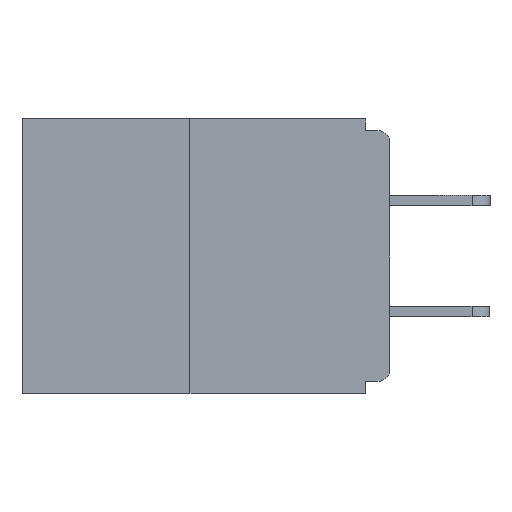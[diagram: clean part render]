
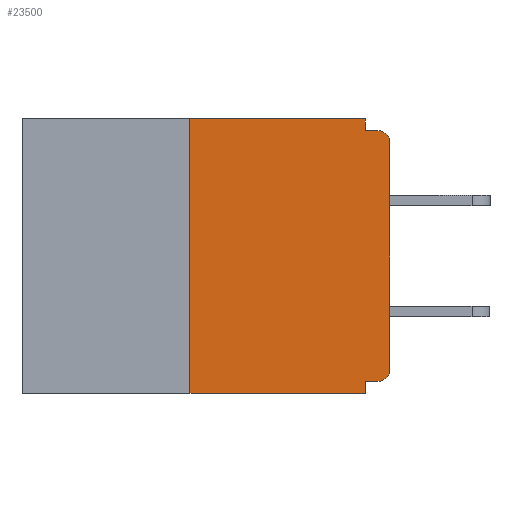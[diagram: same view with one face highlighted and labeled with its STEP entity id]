
A CAD part, left-side view. The second image highlights one B-rep face of the part: STEP entity #23500.
In plain terms, the highlighted planar face has unit normal (-1, 0, 0).
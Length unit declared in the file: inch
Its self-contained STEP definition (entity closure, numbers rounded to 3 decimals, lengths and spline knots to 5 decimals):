
#420 = DIRECTION ( 'NONE',  ( 0., 0., -1. ) ) ;
#530 = AXIS2_PLACEMENT_3D ( 'NONE', #22053, #16932, #420 ) ;
#703 = CARTESIAN_POINT ( 'NONE',  ( 0., 0.015, -0.015 ) ) ;
#951 = DIRECTION ( 'NONE',  ( -1., 0., 0. ) ) ;
#2129 = LINE ( 'NONE', #2693, #16159 ) ;
#2439 = CARTESIAN_POINT ( 'NONE',  ( 0., 0.015, -0.328 ) ) ;
#2693 = CARTESIAN_POINT ( 'NONE',  ( 0., 0.031, 0. ) ) ;
#3044 = EDGE_CURVE ( 'NONE', #8765, #3837, #5856, .T. ) ;
#3158 = LINE ( 'NONE', #17375, #16591 ) ;
#3267 = VERTEX_POINT ( 'NONE', #6853 ) ;
#3383 = CARTESIAN_POINT ( 'NONE',  ( 0., 0., -0.015 ) ) ;
#3719 = CARTESIAN_POINT ( 'NONE',  ( 0., 0.46, -0.343 ) ) ;
#3837 = VERTEX_POINT ( 'NONE', #6579 ) ;
#3854 = EDGE_CURVE ( 'NONE', #17910, #6839, #3158, .T. ) ;
#3873 = FACE_OUTER_BOUND ( 'NONE', #7783, .T. ) ;
#3999 = PLANE ( 'NONE',  #530 ) ;
#4750 = CARTESIAN_POINT ( 'NONE',  ( 0., 0.46, 0. ) ) ;
#5240 = EDGE_CURVE ( 'NONE', #3267, #11360, #7629, .T. ) ;
#5808 = DIRECTION ( 'NONE',  ( 0., -1., 0. ) ) ;
#5856 = CIRCLE ( 'NONE', #20190, 0.015 ) ;
#5893 = ORIENTED_EDGE ( 'NONE', *, *, #5240, .F. ) ;
#6246 = ORIENTED_EDGE ( 'NONE', *, *, #3854, .F. ) ;
#6266 = VERTEX_POINT ( 'NONE', #19514 ) ;
#6411 = DIRECTION ( 'NONE',  ( 0., 0., 1. ) ) ;
#6579 = CARTESIAN_POINT ( 'NONE',  ( 0., 0., -0.313 ) ) ;
#6693 = VECTOR ( 'NONE', #16427, 39.37008 ) ;
#6839 = VERTEX_POINT ( 'NONE', #11793 ) ;
#6853 = CARTESIAN_POINT ( 'NONE',  ( 0., 0.031, -0.328 ) ) ;
#7018 = ORIENTED_EDGE ( 'NONE', *, *, #14868, .F. ) ;
#7549 = VECTOR ( 'NONE', #11493, 39.37008 ) ;
#7560 = AXIS2_PLACEMENT_3D ( 'NONE', #17257, #951, #20951 ) ;
#7629 = LINE ( 'NONE', #14962, #16805 ) ;
#7660 = EDGE_CURVE ( 'NONE', #3837, #6266, #22146, .T. ) ;
#7686 = EDGE_CURVE ( 'NONE', #15214, #12911, #2129, .T. ) ;
#7783 = EDGE_LOOP ( 'NONE', ( #7018, #6246, #10575, #5893, #18327, #8255, #22566, #16024, #8651, #13697 ) ) ;
#7899 = EDGE_CURVE ( 'NONE', #17910, #11360, #10119, .T. ) ;
#8255 = ORIENTED_EDGE ( 'NONE', *, *, #3044, .T. ) ;
#8651 = ORIENTED_EDGE ( 'NONE', *, *, #9510, .F. ) ;
#8711 = LINE ( 'NONE', #4750, #22399 ) ;
#8765 = VERTEX_POINT ( 'NONE', #2439 ) ;
#9075 = LINE ( 'NONE', #13801, #19060 ) ;
#9510 = EDGE_CURVE ( 'NONE', #12911, #14709, #19957, .T. ) ;
#9828 = CARTESIAN_POINT ( 'NONE',  ( 0., 0.031, 0. ) ) ;
#10119 = LINE ( 'NONE', #3719, #6693 ) ;
#10575 = ORIENTED_EDGE ( 'NONE', *, *, #7899, .T. ) ;
#11287 = CARTESIAN_POINT ( 'NONE',  ( 0., 0.031, -0.015 ) ) ;
#11360 = VERTEX_POINT ( 'NONE', #12148 ) ;
#11493 = DIRECTION ( 'NONE',  ( 0., 0., 1. ) ) ;
#11589 = VECTOR ( 'NONE', #16171, 39.37008 ) ;
#11793 = CARTESIAN_POINT ( 'NONE',  ( 0., 0.25, 0. ) ) ;
#12148 = CARTESIAN_POINT ( 'NONE',  ( 0., 0.031, -0.343 ) ) ;
#12911 = VERTEX_POINT ( 'NONE', #11287 ) ;
#13697 = ORIENTED_EDGE ( 'NONE', *, *, #7686, .F. ) ;
#13801 = CARTESIAN_POINT ( 'NONE',  ( 0., 0., -0.328 ) ) ;
#14533 = CARTESIAN_POINT ( 'NONE',  ( 0., 0.015, -0.313 ) ) ;
#14709 = VERTEX_POINT ( 'NONE', #703 ) ;
#14868 = EDGE_CURVE ( 'NONE', #6839, #15214, #8711, .T. ) ;
#14962 = CARTESIAN_POINT ( 'NONE',  ( 0., 0.031, -0.343 ) ) ;
#15214 = VERTEX_POINT ( 'NONE', #9828 ) ;
#15376 = EDGE_CURVE ( 'NONE', #6266, #14709, #18694, .T. ) ;
#15517 = DIRECTION ( 'NONE',  ( 0., 0., -1. ) ) ;
#16024 = ORIENTED_EDGE ( 'NONE', *, *, #15376, .T. ) ;
#16159 = VECTOR ( 'NONE', #15517, 39.37008 ) ;
#16171 = DIRECTION ( 'NONE',  ( 0., -1., 0. ) ) ;
#16427 = DIRECTION ( 'NONE',  ( 0., -1., 0. ) ) ;
#16460 = DIRECTION ( 'NONE',  ( 0., 0., -1. ) ) ;
#16591 = VECTOR ( 'NONE', #6411, 39.37008 ) ;
#16805 = VECTOR ( 'NONE', #16460, 39.37008 ) ;
#16932 = DIRECTION ( 'NONE',  ( 1., 0., 0. ) ) ;
#17257 = CARTESIAN_POINT ( 'NONE',  ( 0., 0.015, -0.03 ) ) ;
#17375 = CARTESIAN_POINT ( 'NONE',  ( 0., 0.25, 0. ) ) ;
#17910 = VERTEX_POINT ( 'NONE', #19260 ) ;
#18327 = ORIENTED_EDGE ( 'NONE', *, *, #22441, .F. ) ;
#18694 = CIRCLE ( 'NONE', #7560, 0.015 ) ;
#19060 = VECTOR ( 'NONE', #22631, 39.37008 ) ;
#19260 = CARTESIAN_POINT ( 'NONE',  ( 0., 0.25, -0.343 ) ) ;
#19514 = CARTESIAN_POINT ( 'NONE',  ( 0., 0., -0.03 ) ) ;
#19957 = LINE ( 'NONE', #3383, #11589 ) ;
#20190 = AXIS2_PLACEMENT_3D ( 'NONE', #14533, #23544, #23464 ) ;
#20947 = CARTESIAN_POINT ( 'NONE',  ( 0., 0., 0. ) ) ;
#20951 = DIRECTION ( 'NONE',  ( 0., 0., -1. ) ) ;
#22053 = CARTESIAN_POINT ( 'NONE',  ( 0., 0.46, 0. ) ) ;
#22146 = LINE ( 'NONE', #20947, #7549 ) ;
#22399 = VECTOR ( 'NONE', #5808, 39.37008 ) ;
#22441 = EDGE_CURVE ( 'NONE', #8765, #3267, #9075, .T. ) ;
#22566 = ORIENTED_EDGE ( 'NONE', *, *, #7660, .T. ) ;
#22631 = DIRECTION ( 'NONE',  ( 0., 1., 0. ) ) ;
#23464 = DIRECTION ( 'NONE',  ( 0., 0., -1. ) ) ;
#23500 = ADVANCED_FACE ( 'NONE', ( #3873 ), #3999, .F. ) ;
#23544 = DIRECTION ( 'NONE',  ( -1., 0., 0. ) ) ;
